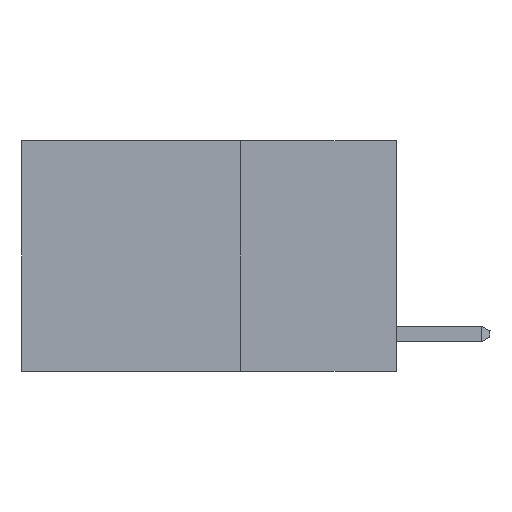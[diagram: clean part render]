
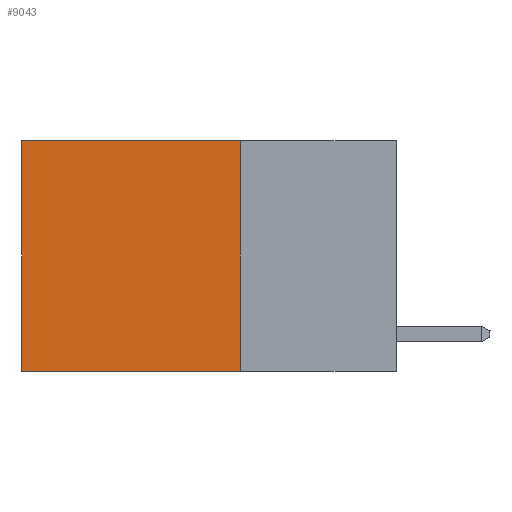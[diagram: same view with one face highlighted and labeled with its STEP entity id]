
A CAD part, left-side view. The second image highlights one B-rep face of the part: STEP entity #9043.
In plain terms, the highlighted planar face has unit normal (-1, 0, 0).
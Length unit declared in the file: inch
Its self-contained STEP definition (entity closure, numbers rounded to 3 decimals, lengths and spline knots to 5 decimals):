
#208 = DIRECTION ( 'NONE',  ( 1., 0., 0. ) ) ;
#995 = VECTOR ( 'NONE', #6840, 39.37008 ) ;
#1163 = LINE ( 'NONE', #1340, #995 ) ;
#1340 = CARTESIAN_POINT ( 'NONE',  ( 0.2625, 0.25, -0.37 ) ) ;
#1544 = CARTESIAN_POINT ( 'NONE',  ( 0.2625, 0.25, 0. ) ) ;
#1636 = DIRECTION ( 'NONE',  ( 0., 0., -1. ) ) ;
#2501 = EDGE_CURVE ( 'NONE', #4440, #8030, #7045, .T. ) ;
#3081 = FACE_OUTER_BOUND ( 'NONE', #9840, .T. ) ;
#3241 = CARTESIAN_POINT ( 'NONE',  ( 0.2625, 0.25, 0. ) ) ;
#4095 = EDGE_CURVE ( 'NONE', #16470, #12821, #14011, .T. ) ;
#4440 = VERTEX_POINT ( 'NONE', #10828 ) ;
#4984 = ORIENTED_EDGE ( 'NONE', *, *, #16745, .F. ) ;
#6840 = DIRECTION ( 'NONE',  ( 0., 1., 0. ) ) ;
#7045 = LINE ( 'NONE', #11125, #9546 ) ;
#7932 = CARTESIAN_POINT ( 'NONE',  ( 0.2625, 0.6, -0.37 ) ) ;
#8030 = VERTEX_POINT ( 'NONE', #7932 ) ;
#8593 = PLANE ( 'NONE',  #17185 ) ;
#8862 = EDGE_CURVE ( 'NONE', #16470, #4440, #13397, .T. ) ;
#9043 = ADVANCED_FACE ( 'NONE', ( #3081 ), #8593, .F. ) ;
#9224 = DIRECTION ( 'NONE',  ( 0., 1., 0. ) ) ;
#9546 = VECTOR ( 'NONE', #16892, 39.37008 ) ;
#9840 = EDGE_LOOP ( 'NONE', ( #12411, #4984, #15958, #14502 ) ) ;
#10238 = CARTESIAN_POINT ( 'NONE',  ( 0.2625, 0.25, -0.37 ) ) ;
#10828 = CARTESIAN_POINT ( 'NONE',  ( 0.2625, 0.6, 0. ) ) ;
#11125 = CARTESIAN_POINT ( 'NONE',  ( 0.2625, 0.6, 0. ) ) ;
#12411 = ORIENTED_EDGE ( 'NONE', *, *, #2501, .T. ) ;
#12821 = VERTEX_POINT ( 'NONE', #10238 ) ;
#13047 = VECTOR ( 'NONE', #9224, 39.37008 ) ;
#13397 = LINE ( 'NONE', #14843, #13047 ) ;
#13506 = VECTOR ( 'NONE', #1636, 39.37008 ) ;
#14011 = LINE ( 'NONE', #1544, #13506 ) ;
#14111 = DIRECTION ( 'NONE',  ( 0., 0., -1. ) ) ;
#14502 = ORIENTED_EDGE ( 'NONE', *, *, #8862, .T. ) ;
#14843 = CARTESIAN_POINT ( 'NONE',  ( 0.2625, 0.25, 0. ) ) ;
#15958 = ORIENTED_EDGE ( 'NONE', *, *, #4095, .F. ) ;
#16470 = VERTEX_POINT ( 'NONE', #3241 ) ;
#16636 = CARTESIAN_POINT ( 'NONE',  ( 0.2625, 0.25, 0. ) ) ;
#16745 = EDGE_CURVE ( 'NONE', #12821, #8030, #1163, .T. ) ;
#16892 = DIRECTION ( 'NONE',  ( 0., 0., -1. ) ) ;
#17185 = AXIS2_PLACEMENT_3D ( 'NONE', #16636, #208, #14111 ) ;
